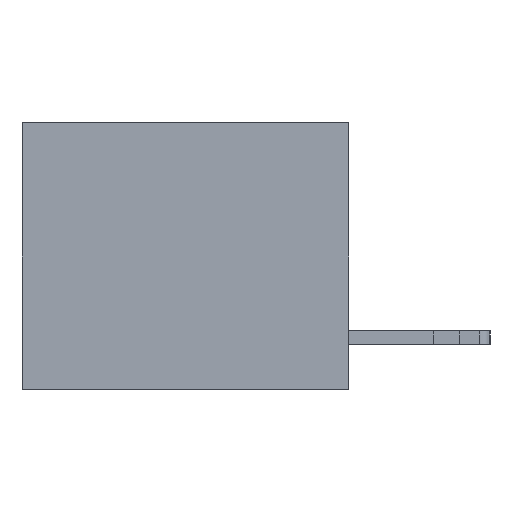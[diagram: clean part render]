
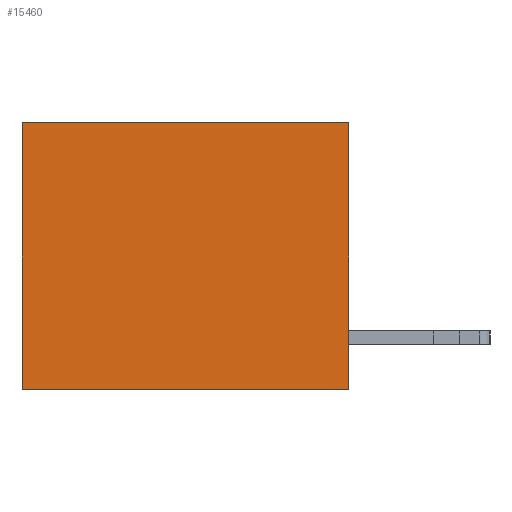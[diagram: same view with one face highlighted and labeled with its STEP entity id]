
A CAD part, left-side view. The second image highlights one B-rep face of the part: STEP entity #15460.
In plain terms, the highlighted planar face has unit normal (-1, 0, 0).
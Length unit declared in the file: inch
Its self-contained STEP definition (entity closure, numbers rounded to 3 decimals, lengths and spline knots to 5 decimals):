
#20 = VECTOR ( 'NONE', #12877, 39.37008 ) ;
#582 = VECTOR ( 'NONE', #11313, 39.37008 ) ;
#2020 = LINE ( 'NONE', #2220, #15339 ) ;
#2220 = CARTESIAN_POINT ( 'NONE',  ( 0.3165, 0., 0. ) ) ;
#2608 = CARTESIAN_POINT ( 'NONE',  ( 0.3165, 0.6, -0.49 ) ) ;
#2845 = FACE_OUTER_BOUND ( 'NONE', #10097, .T. ) ;
#3933 = CARTESIAN_POINT ( 'NONE',  ( 0.3165, 0., -0.49 ) ) ;
#4053 = DIRECTION ( 'NONE',  ( 1., 0., 0. ) ) ;
#4312 = CARTESIAN_POINT ( 'NONE',  ( 0.3165, 0., 0. ) ) ;
#4358 = CARTESIAN_POINT ( 'NONE',  ( 0.3165, 0., -0.49 ) ) ;
#4912 = EDGE_CURVE ( 'NONE', #11212, #5872, #2020, .T. ) ;
#5530 = DIRECTION ( 'NONE',  ( 0., 0., -1. ) ) ;
#5574 = LINE ( 'NONE', #4358, #7614 ) ;
#5588 = CARTESIAN_POINT ( 'NONE',  ( 0.3165, 0., -0.49 ) ) ;
#5872 = VERTEX_POINT ( 'NONE', #18975 ) ;
#7538 = ORIENTED_EDGE ( 'NONE', *, *, #16557, .F. ) ;
#7614 = VECTOR ( 'NONE', #14598, 39.37008 ) ;
#8408 = PLANE ( 'NONE',  #13512 ) ;
#8418 = LINE ( 'NONE', #3933, #582 ) ;
#9630 = ORIENTED_EDGE ( 'NONE', *, *, #13362, .F. ) ;
#10097 = EDGE_LOOP ( 'NONE', ( #12912, #7538, #9630, #18619 ) ) ;
#11136 = DIRECTION ( 'NONE',  ( 0., 1., 0. ) ) ;
#11212 = VERTEX_POINT ( 'NONE', #4312 ) ;
#11270 = VERTEX_POINT ( 'NONE', #17717 ) ;
#11313 = DIRECTION ( 'NONE',  ( 0., 1., 0. ) ) ;
#12596 = VERTEX_POINT ( 'NONE', #18644 ) ;
#12877 = DIRECTION ( 'NONE',  ( 0., 0., -1. ) ) ;
#12912 = ORIENTED_EDGE ( 'NONE', *, *, #18953, .T. ) ;
#13362 = EDGE_CURVE ( 'NONE', #11212, #11270, #5574, .T. ) ;
#13512 = AXIS2_PLACEMENT_3D ( 'NONE', #5588, #4053, #5530 ) ;
#14518 = LINE ( 'NONE', #2608, #20 ) ;
#14598 = DIRECTION ( 'NONE',  ( 0., 0., -1. ) ) ;
#15339 = VECTOR ( 'NONE', #11136, 39.37008 ) ;
#15460 = ADVANCED_FACE ( 'NONE', ( #2845 ), #8408, .F. ) ;
#16557 = EDGE_CURVE ( 'NONE', #11270, #12596, #8418, .T. ) ;
#17717 = CARTESIAN_POINT ( 'NONE',  ( 0.3165, 0., -0.49 ) ) ;
#18619 = ORIENTED_EDGE ( 'NONE', *, *, #4912, .T. ) ;
#18644 = CARTESIAN_POINT ( 'NONE',  ( 0.3165, 0.6, -0.49 ) ) ;
#18953 = EDGE_CURVE ( 'NONE', #5872, #12596, #14518, .T. ) ;
#18975 = CARTESIAN_POINT ( 'NONE',  ( 0.3165, 0.6, 0. ) ) ;
